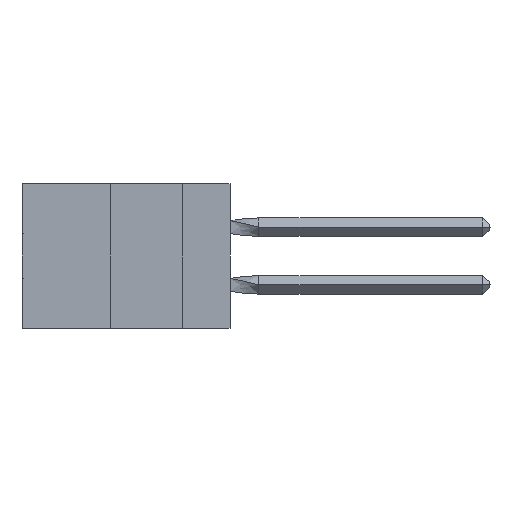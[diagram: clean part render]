
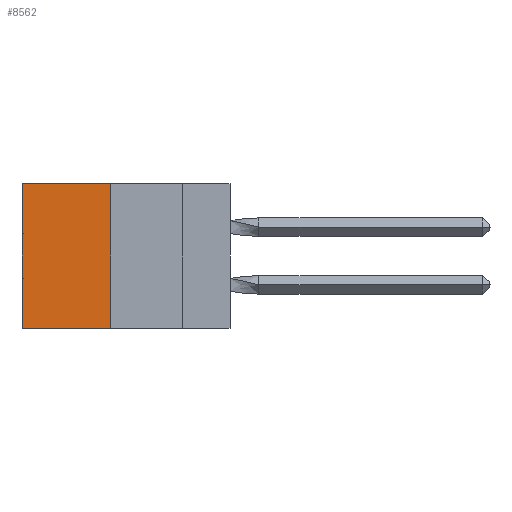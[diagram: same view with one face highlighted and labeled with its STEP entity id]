
A CAD part, left-side view. The second image highlights one B-rep face of the part: STEP entity #8562.
In plain terms, the highlighted planar face has unit normal (-1, 0, 0).
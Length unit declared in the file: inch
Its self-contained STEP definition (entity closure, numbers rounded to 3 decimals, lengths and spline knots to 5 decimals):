
#715 = DIRECTION ( 'NONE',  ( 0., 1., 0. ) ) ;
#1431 = FACE_OUTER_BOUND ( 'NONE', #7410, .T. ) ;
#1748 = VECTOR ( 'NONE', #715, 39.37008 ) ;
#2959 = DIRECTION ( 'NONE',  ( 0., 1., 0. ) ) ;
#3918 = VERTEX_POINT ( 'NONE', #25942 ) ;
#4483 = CARTESIAN_POINT ( 'NONE',  ( 0.305, 0.72, 0. ) ) ;
#5490 = VERTEX_POINT ( 'NONE', #33649 ) ;
#5847 = PLANE ( 'NONE',  #13173 ) ;
#7294 = VERTEX_POINT ( 'NONE', #4483 ) ;
#7410 = EDGE_LOOP ( 'NONE', ( #19684, #29774, #18447, #19851 ) ) ;
#8562 = ADVANCED_FACE ( 'NONE', ( #1431 ), #5847, .F. ) ;
#8820 = LINE ( 'NONE', #10746, #21228 ) ;
#9105 = EDGE_CURVE ( 'NONE', #7294, #5490, #18801, .T. ) ;
#10746 = CARTESIAN_POINT ( 'NONE',  ( 0.305, 0.413, -0.5 ) ) ;
#11211 = EDGE_CURVE ( 'NONE', #24100, #3918, #8820, .T. ) ;
#13053 = DIRECTION ( 'NONE',  ( 1., 0., 0. ) ) ;
#13173 = AXIS2_PLACEMENT_3D ( 'NONE', #15804, #13053, #20275 ) ;
#15312 = CARTESIAN_POINT ( 'NONE',  ( 0.305, 0.72, -0.5 ) ) ;
#15804 = CARTESIAN_POINT ( 'NONE',  ( 0.305, 0.413, -0.5 ) ) ;
#17831 = DIRECTION ( 'NONE',  ( 0., 0., -1. ) ) ;
#18447 = ORIENTED_EDGE ( 'NONE', *, *, #11211, .F. ) ;
#18801 = LINE ( 'NONE', #15312, #22351 ) ;
#19684 = ORIENTED_EDGE ( 'NONE', *, *, #9105, .T. ) ;
#19851 = ORIENTED_EDGE ( 'NONE', *, *, #40999, .T. ) ;
#20275 = DIRECTION ( 'NONE',  ( 0., 0., -1. ) ) ;
#21228 = VECTOR ( 'NONE', #17831, 39.37008 ) ;
#22351 = VECTOR ( 'NONE', #31349, 39.37008 ) ;
#24100 = VERTEX_POINT ( 'NONE', #26606 ) ;
#25246 = EDGE_CURVE ( 'NONE', #3918, #5490, #25666, .T. ) ;
#25666 = LINE ( 'NONE', #28737, #41485 ) ;
#25942 = CARTESIAN_POINT ( 'NONE',  ( 0.305, 0.413, -0.5 ) ) ;
#26606 = CARTESIAN_POINT ( 'NONE',  ( 0.305, 0.413, 0. ) ) ;
#28737 = CARTESIAN_POINT ( 'NONE',  ( 0.305, 0.413, -0.5 ) ) ;
#29774 = ORIENTED_EDGE ( 'NONE', *, *, #25246, .F. ) ;
#30976 = LINE ( 'NONE', #36821, #1748 ) ;
#31349 = DIRECTION ( 'NONE',  ( 0., 0., -1. ) ) ;
#33649 = CARTESIAN_POINT ( 'NONE',  ( 0.305, 0.72, -0.5 ) ) ;
#36821 = CARTESIAN_POINT ( 'NONE',  ( 0.305, 0.413, 0. ) ) ;
#40999 = EDGE_CURVE ( 'NONE', #24100, #7294, #30976, .T. ) ;
#41485 = VECTOR ( 'NONE', #2959, 39.37008 ) ;
